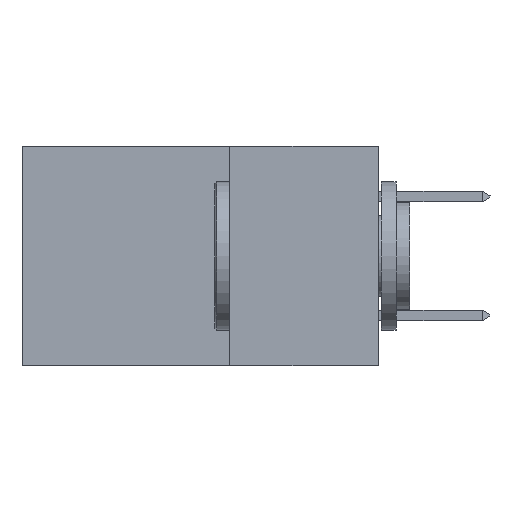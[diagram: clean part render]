
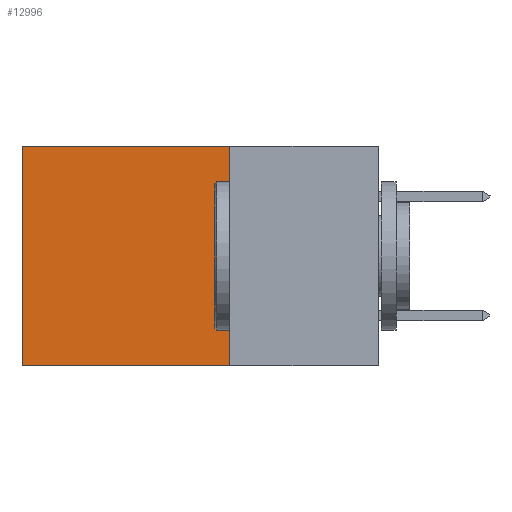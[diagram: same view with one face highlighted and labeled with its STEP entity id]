
A CAD part, left-side view. The second image highlights one B-rep face of the part: STEP entity #12996.
In plain terms, the highlighted planar face has unit normal (-1, 0, 0).
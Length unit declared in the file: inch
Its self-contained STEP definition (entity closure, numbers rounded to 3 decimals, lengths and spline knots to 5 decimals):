
#596 = LINE ( 'NONE', #17758, #1240 ) ;
#1085 = VERTEX_POINT ( 'NONE', #12089 ) ;
#1090 = CARTESIAN_POINT ( 'NONE',  ( 0.2615, 0.25, -0.37 ) ) ;
#1240 = VECTOR ( 'NONE', #19769, 39.37008 ) ;
#2322 = CARTESIAN_POINT ( 'NONE',  ( 0.2615, 0.6, -0.37 ) ) ;
#2604 = VERTEX_POINT ( 'NONE', #2322 ) ;
#3558 = LINE ( 'NONE', #19023, #9887 ) ;
#4282 = ORIENTED_EDGE ( 'NONE', *, *, #20644, .F. ) ;
#4774 = EDGE_CURVE ( 'NONE', #1085, #9862, #596, .T. ) ;
#5728 = ORIENTED_EDGE ( 'NONE', *, *, #17357, .T. ) ;
#7855 = PLANE ( 'NONE',  #9954 ) ;
#9827 = ORIENTED_EDGE ( 'NONE', *, *, #21449, .F. ) ;
#9862 = VERTEX_POINT ( 'NONE', #12420 ) ;
#9887 = VECTOR ( 'NONE', #10748, 39.37008 ) ;
#9954 = AXIS2_PLACEMENT_3D ( 'NONE', #1090, #21513, #13008 ) ;
#10738 = DIRECTION ( 'NONE',  ( 0., 0., -1. ) ) ;
#10748 = DIRECTION ( 'NONE',  ( 0., 1., 0. ) ) ;
#11400 = DIRECTION ( 'NONE',  ( 0., 0., -1. ) ) ;
#12089 = CARTESIAN_POINT ( 'NONE',  ( 0.2615, 0.25, 0. ) ) ;
#12420 = CARTESIAN_POINT ( 'NONE',  ( 0.2615, 0.6, 0. ) ) ;
#12996 = ADVANCED_FACE ( 'NONE', ( #18027 ), #7855, .F. ) ;
#13008 = DIRECTION ( 'NONE',  ( 0., 0., -1. ) ) ;
#13277 = CARTESIAN_POINT ( 'NONE',  ( 0.2615, 0.25, -0.37 ) ) ;
#14801 = VECTOR ( 'NONE', #10738, 39.37008 ) ;
#15645 = VECTOR ( 'NONE', #11400, 39.37008 ) ;
#17357 = EDGE_CURVE ( 'NONE', #9862, #2604, #17984, .T. ) ;
#17758 = CARTESIAN_POINT ( 'NONE',  ( 0.2615, 0.25, 0. ) ) ;
#17984 = LINE ( 'NONE', #19239, #14801 ) ;
#18027 = FACE_OUTER_BOUND ( 'NONE', #20686, .T. ) ;
#19023 = CARTESIAN_POINT ( 'NONE',  ( 0.2615, 0.25, -0.37 ) ) ;
#19239 = CARTESIAN_POINT ( 'NONE',  ( 0.2615, 0.6, -0.37 ) ) ;
#19573 = ORIENTED_EDGE ( 'NONE', *, *, #4774, .T. ) ;
#19769 = DIRECTION ( 'NONE',  ( 0., 1., 0. ) ) ;
#20644 = EDGE_CURVE ( 'NONE', #22075, #2604, #3558, .T. ) ;
#20686 = EDGE_LOOP ( 'NONE', ( #5728, #4282, #9827, #19573 ) ) ;
#20713 = CARTESIAN_POINT ( 'NONE',  ( 0.2615, 0.25, -0.37 ) ) ;
#21449 = EDGE_CURVE ( 'NONE', #1085, #22075, #21801, .T. ) ;
#21513 = DIRECTION ( 'NONE',  ( 1., 0., 0. ) ) ;
#21801 = LINE ( 'NONE', #13277, #15645 ) ;
#22075 = VERTEX_POINT ( 'NONE', #20713 ) ;
